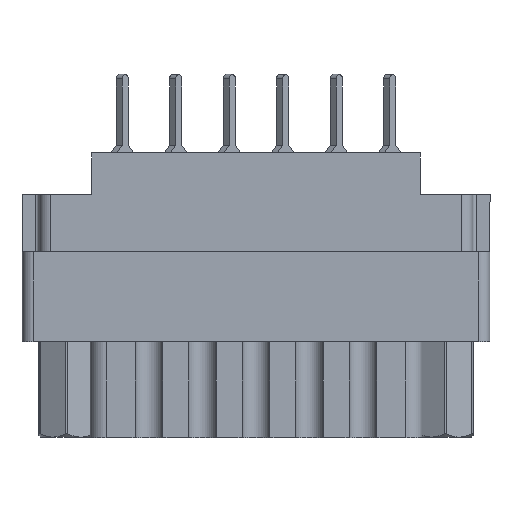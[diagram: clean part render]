
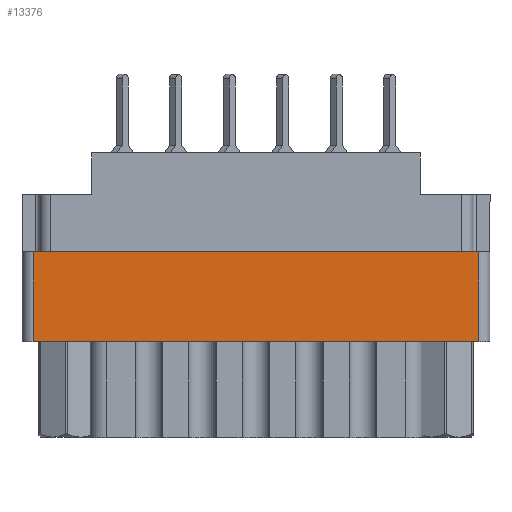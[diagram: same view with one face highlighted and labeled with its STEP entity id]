
A CAD part, front view. The second image highlights one B-rep face of the part: STEP entity #13376.
In plain terms, the highlighted planar face has unit normal (0, -1, 0).
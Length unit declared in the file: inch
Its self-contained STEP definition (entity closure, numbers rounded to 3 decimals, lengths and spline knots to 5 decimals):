
#398 = DIRECTION ( 'NONE',  ( 0., 0., -1. ) ) ;
#809 = EDGE_CURVE ( 'NONE', #3968, #30441, #8417, .T. ) ;
#901 = EDGE_CURVE ( 'NONE', #12971, #12879, #6430, .T. ) ;
#1024 = CARTESIAN_POINT ( 'NONE',  ( 0.624, -0.343, -0.529 ) ) ;
#1931 = LINE ( 'NONE', #19482, #29622 ) ;
#2965 = EDGE_CURVE ( 'NONE', #3968, #12879, #19318, .T. ) ;
#3345 = PLANE ( 'NONE',  #5634 ) ;
#3968 = VERTEX_POINT ( 'NONE', #25266 ) ;
#4241 = DIRECTION ( 'NONE',  ( 0., 0., 1. ) ) ;
#5634 = AXIS2_PLACEMENT_3D ( 'NONE', #28286, #25338, #398 ) ;
#5741 = ORIENTED_EDGE ( 'NONE', *, *, #901, .F. ) ;
#5802 = CARTESIAN_POINT ( 'NONE',  ( 0.624, -0.343, -0.277 ) ) ;
#5920 = CARTESIAN_POINT ( 'NONE',  ( -0.624, -0.343, -0.277 ) ) ;
#6430 = LINE ( 'NONE', #20882, #21385 ) ;
#6601 = DIRECTION ( 'NONE',  ( -1., 0., 0. ) ) ;
#8417 = LINE ( 'NONE', #1024, #15626 ) ;
#8961 = ORIENTED_EDGE ( 'NONE', *, *, #809, .F. ) ;
#11008 = CARTESIAN_POINT ( 'NONE',  ( -0.624, -0.343, -0.529 ) ) ;
#12879 = VERTEX_POINT ( 'NONE', #5802 ) ;
#12971 = VERTEX_POINT ( 'NONE', #5920 ) ;
#13355 = DIRECTION ( 'NONE',  ( 0., 0., 1. ) ) ;
#13376 = ADVANCED_FACE ( 'NONE', ( #30269 ), #3345, .T. ) ;
#14236 = VECTOR ( 'NONE', #13355, 39.37008 ) ;
#15626 = VECTOR ( 'NONE', #6601, 39.37008 ) ;
#19318 = LINE ( 'NONE', #28125, #14236 ) ;
#19482 = CARTESIAN_POINT ( 'NONE',  ( -0.624, -0.343, -0.798 ) ) ;
#20882 = CARTESIAN_POINT ( 'NONE',  ( -0.656, -0.343, -0.277 ) ) ;
#21385 = VECTOR ( 'NONE', #28737, 39.37008 ) ;
#22902 = EDGE_CURVE ( 'NONE', #30441, #12971, #1931, .T. ) ;
#23610 = ORIENTED_EDGE ( 'NONE', *, *, #2965, .T. ) ;
#24706 = ORIENTED_EDGE ( 'NONE', *, *, #22902, .F. ) ;
#25266 = CARTESIAN_POINT ( 'NONE',  ( 0.624, -0.343, -0.529 ) ) ;
#25311 = EDGE_LOOP ( 'NONE', ( #24706, #8961, #23610, #5741 ) ) ;
#25338 = DIRECTION ( 'NONE',  ( 0., -1., 0. ) ) ;
#28125 = CARTESIAN_POINT ( 'NONE',  ( 0.624, -0.343, -0.798 ) ) ;
#28286 = CARTESIAN_POINT ( 'NONE',  ( -0.624, -0.343, -0.798 ) ) ;
#28737 = DIRECTION ( 'NONE',  ( 1., 0., 0. ) ) ;
#29622 = VECTOR ( 'NONE', #4241, 39.37008 ) ;
#30269 = FACE_OUTER_BOUND ( 'NONE', #25311, .T. ) ;
#30441 = VERTEX_POINT ( 'NONE', #11008 ) ;
